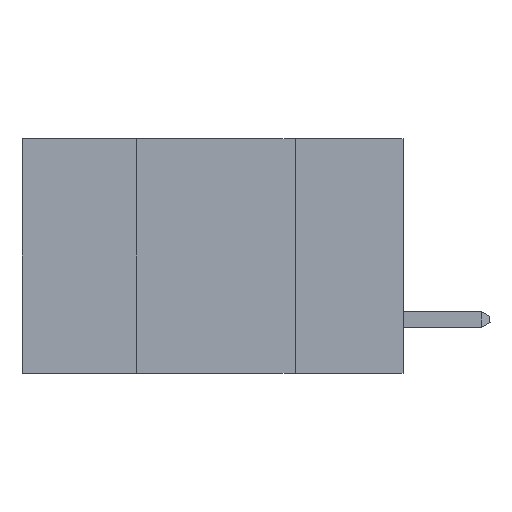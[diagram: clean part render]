
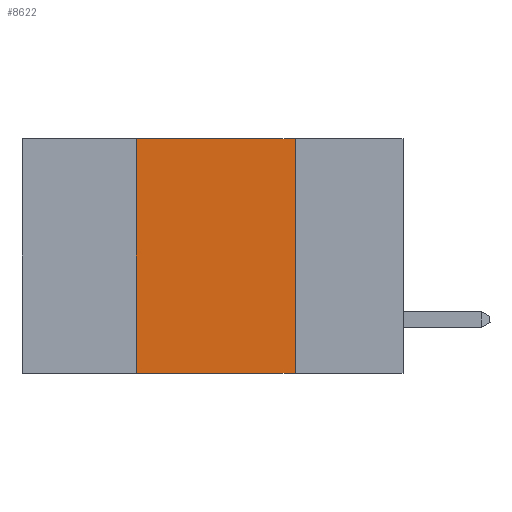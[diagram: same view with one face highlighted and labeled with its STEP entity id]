
A CAD part, left-side view. The second image highlights one B-rep face of the part: STEP entity #8622.
In plain terms, the highlighted planar face has unit normal (-1, 0, 0).
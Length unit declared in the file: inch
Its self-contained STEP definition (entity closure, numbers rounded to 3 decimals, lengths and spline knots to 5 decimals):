
#407 = CARTESIAN_POINT ( 'NONE',  ( 0., 0.17, 0. ) ) ;
#513 = DIRECTION ( 'NONE',  ( 0., 0., -1. ) ) ;
#516 = EDGE_LOOP ( 'NONE', ( #2606, #1094, #8797, #3895 ) ) ;
#1094 = ORIENTED_EDGE ( 'NONE', *, *, #7820, .F. ) ;
#1878 = FACE_OUTER_BOUND ( 'NONE', #516, .T. ) ;
#1948 = CARTESIAN_POINT ( 'NONE',  ( 0., 0.6, 0. ) ) ;
#2152 = CARTESIAN_POINT ( 'NONE',  ( 0., 0.17, -0.37 ) ) ;
#2236 = VECTOR ( 'NONE', #7036, 39.37008 ) ;
#2423 = VERTEX_POINT ( 'NONE', #2152 ) ;
#2606 = ORIENTED_EDGE ( 'NONE', *, *, #2834, .F. ) ;
#2637 = CARTESIAN_POINT ( 'NONE',  ( 0., 0.17, 0. ) ) ;
#2834 = EDGE_CURVE ( 'NONE', #3836, #2423, #3271, .T. ) ;
#3265 = CARTESIAN_POINT ( 'NONE',  ( 0., 0.6, 0. ) ) ;
#3271 = LINE ( 'NONE', #407, #2236 ) ;
#3472 = DIRECTION ( 'NONE',  ( 0., -1., 0. ) ) ;
#3509 = DIRECTION ( 'NONE',  ( 0., 0., 1. ) ) ;
#3836 = VERTEX_POINT ( 'NONE', #2637 ) ;
#3868 = CARTESIAN_POINT ( 'NONE',  ( 0., 0.42, 0. ) ) ;
#3895 = ORIENTED_EDGE ( 'NONE', *, *, #4815, .T. ) ;
#4068 = VECTOR ( 'NONE', #3509, 39.37008 ) ;
#4207 = CARTESIAN_POINT ( 'NONE',  ( 0., 0.42, 0. ) ) ;
#4542 = LINE ( 'NONE', #4207, #4068 ) ;
#4608 = LINE ( 'NONE', #8416, #8315 ) ;
#4626 = AXIS2_PLACEMENT_3D ( 'NONE', #3265, #7142, #513 ) ;
#4815 = EDGE_CURVE ( 'NONE', #6529, #2423, #4608, .T. ) ;
#5447 = PLANE ( 'NONE',  #4626 ) ;
#6208 = LINE ( 'NONE', #1948, #7130 ) ;
#6346 = VERTEX_POINT ( 'NONE', #3868 ) ;
#6529 = VERTEX_POINT ( 'NONE', #7722 ) ;
#6864 = DIRECTION ( 'NONE',  ( 0., -1., 0. ) ) ;
#7036 = DIRECTION ( 'NONE',  ( 0., 0., -1. ) ) ;
#7130 = VECTOR ( 'NONE', #3472, 39.37008 ) ;
#7142 = DIRECTION ( 'NONE',  ( 1., 0., 0. ) ) ;
#7691 = EDGE_CURVE ( 'NONE', #6529, #6346, #4542, .T. ) ;
#7722 = CARTESIAN_POINT ( 'NONE',  ( 0., 0.42, -0.37 ) ) ;
#7820 = EDGE_CURVE ( 'NONE', #6346, #3836, #6208, .T. ) ;
#8315 = VECTOR ( 'NONE', #6864, 39.37008 ) ;
#8416 = CARTESIAN_POINT ( 'NONE',  ( 0., 0.6, -0.37 ) ) ;
#8622 = ADVANCED_FACE ( 'NONE', ( #1878 ), #5447, .F. ) ;
#8797 = ORIENTED_EDGE ( 'NONE', *, *, #7691, .F. ) ;
